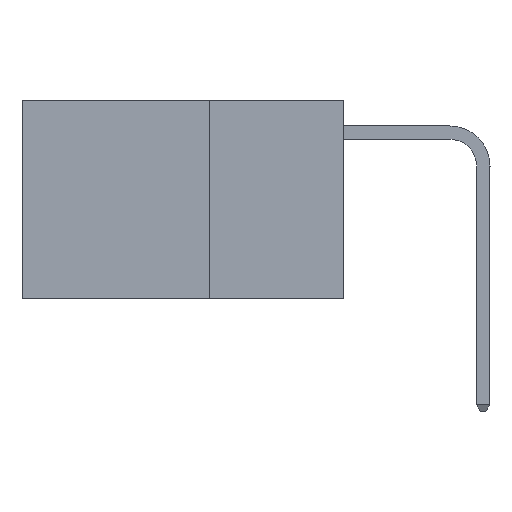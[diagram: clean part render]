
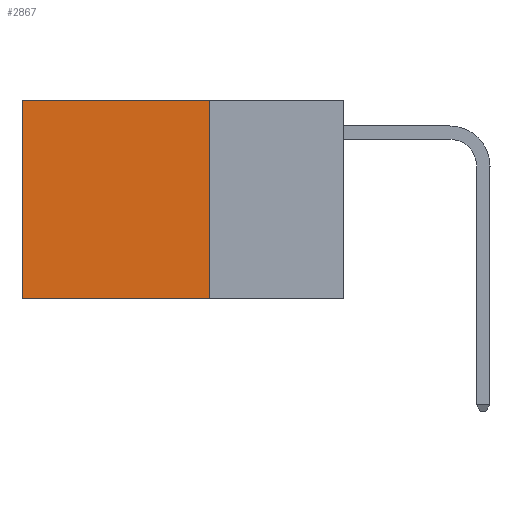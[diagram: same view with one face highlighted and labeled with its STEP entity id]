
A CAD part, left-side view. The second image highlights one B-rep face of the part: STEP entity #2867.
In plain terms, the highlighted planar face has unit normal (-1, 0, 0).
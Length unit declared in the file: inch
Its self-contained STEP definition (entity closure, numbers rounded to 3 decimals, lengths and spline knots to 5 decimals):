
#187 = DIRECTION ( 'NONE',  ( 0., 1., 0. ) ) ;
#271 = CARTESIAN_POINT ( 'NONE',  ( 0.2625, 0.6, 0. ) ) ;
#702 = ORIENTED_EDGE ( 'NONE', *, *, #2681, .T. ) ;
#823 = ORIENTED_EDGE ( 'NONE', *, *, #1927, .F. ) ;
#1131 = VERTEX_POINT ( 'NONE', #6221 ) ;
#1173 = DIRECTION ( 'NONE',  ( 0., 0., -1. ) ) ;
#1588 = VECTOR ( 'NONE', #3965, 39.37008 ) ;
#1622 = LINE ( 'NONE', #6923, #1588 ) ;
#1825 = CARTESIAN_POINT ( 'NONE',  ( 0.2625, 0.25, 0. ) ) ;
#1927 = EDGE_CURVE ( 'NONE', #8443, #7741, #1622, .T. ) ;
#2681 = EDGE_CURVE ( 'NONE', #4574, #1131, #8485, .T. ) ;
#2867 = ADVANCED_FACE ( 'NONE', ( #7151 ), #9999, .F. ) ;
#3138 = VECTOR ( 'NONE', #1173, 39.37008 ) ;
#3292 = CARTESIAN_POINT ( 'NONE',  ( 0.2625, 0.25, 0. ) ) ;
#3472 = CARTESIAN_POINT ( 'NONE',  ( 0.2625, 0.25, 0. ) ) ;
#3728 = DIRECTION ( 'NONE',  ( 1., 0., 0. ) ) ;
#3965 = DIRECTION ( 'NONE',  ( 0., 1., 0. ) ) ;
#4574 = VERTEX_POINT ( 'NONE', #3292 ) ;
#4792 = VECTOR ( 'NONE', #8779, 39.37008 ) ;
#5127 = AXIS2_PLACEMENT_3D ( 'NONE', #1825, #3728, #7545 ) ;
#5336 = LINE ( 'NONE', #271, #3138 ) ;
#5859 = EDGE_CURVE ( 'NONE', #4574, #8443, #9221, .T. ) ;
#6104 = CARTESIAN_POINT ( 'NONE',  ( 0.2625, 0.6, -0.37 ) ) ;
#6221 = CARTESIAN_POINT ( 'NONE',  ( 0.2625, 0.6, 0. ) ) ;
#6923 = CARTESIAN_POINT ( 'NONE',  ( 0.2625, 0.25, -0.37 ) ) ;
#7151 = FACE_OUTER_BOUND ( 'NONE', #9985, .T. ) ;
#7545 = DIRECTION ( 'NONE',  ( 0., 0., -1. ) ) ;
#7741 = VERTEX_POINT ( 'NONE', #6104 ) ;
#8074 = CARTESIAN_POINT ( 'NONE',  ( 0.2625, 0.25, -0.37 ) ) ;
#8443 = VERTEX_POINT ( 'NONE', #8074 ) ;
#8485 = LINE ( 'NONE', #8970, #10578 ) ;
#8700 = ORIENTED_EDGE ( 'NONE', *, *, #9396, .T. ) ;
#8720 = ORIENTED_EDGE ( 'NONE', *, *, #5859, .F. ) ;
#8779 = DIRECTION ( 'NONE',  ( 0., 0., -1. ) ) ;
#8970 = CARTESIAN_POINT ( 'NONE',  ( 0.2625, 0.25, 0. ) ) ;
#9221 = LINE ( 'NONE', #3472, #4792 ) ;
#9396 = EDGE_CURVE ( 'NONE', #1131, #7741, #5336, .T. ) ;
#9985 = EDGE_LOOP ( 'NONE', ( #8700, #823, #8720, #702 ) ) ;
#9999 = PLANE ( 'NONE',  #5127 ) ;
#10578 = VECTOR ( 'NONE', #187, 39.37008 ) ;
